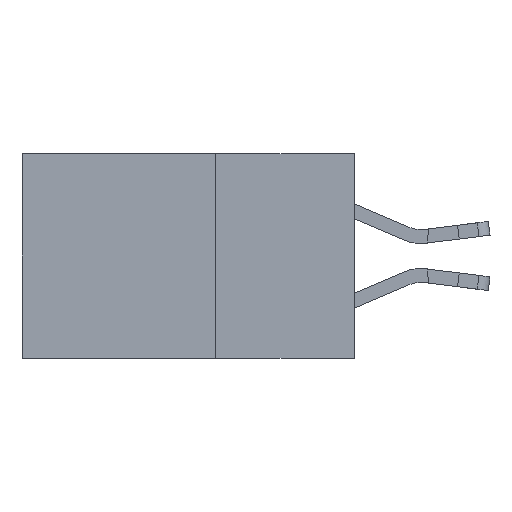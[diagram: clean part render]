
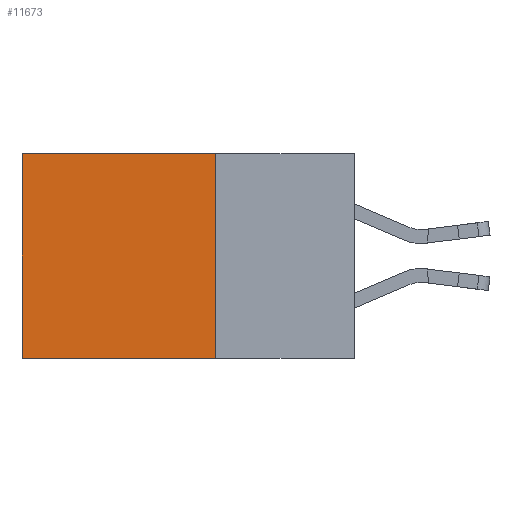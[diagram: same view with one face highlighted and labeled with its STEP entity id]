
A CAD part, left-side view. The second image highlights one B-rep face of the part: STEP entity #11673.
In plain terms, the highlighted planar face has unit normal (-1, 0, 0).
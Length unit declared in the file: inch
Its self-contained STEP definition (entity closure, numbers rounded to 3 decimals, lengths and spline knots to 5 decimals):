
#77 = VECTOR ( 'NONE', #8197, 39.37008 ) ;
#394 = LINE ( 'NONE', #10285, #77 ) ;
#401 = ORIENTED_EDGE ( 'NONE', *, *, #12165, .T. ) ;
#487 = DIRECTION ( 'NONE',  ( 0., 0., -1. ) ) ;
#513 = CARTESIAN_POINT ( 'NONE',  ( 0.298, 0.6, -0.37 ) ) ;
#648 = VERTEX_POINT ( 'NONE', #13406 ) ;
#827 = CARTESIAN_POINT ( 'NONE',  ( 0.298, 0.25, -0.37 ) ) ;
#1503 = LINE ( 'NONE', #11725, #6780 ) ;
#2200 = LINE ( 'NONE', #4501, #4677 ) ;
#2387 = DIRECTION ( 'NONE',  ( 0., 1., 0. ) ) ;
#2660 = VECTOR ( 'NONE', #4953, 39.37008 ) ;
#2956 = CARTESIAN_POINT ( 'NONE',  ( 0.298, 0.6, 0. ) ) ;
#3911 = CARTESIAN_POINT ( 'NONE',  ( 0.298, 0.6, 0. ) ) ;
#4501 = CARTESIAN_POINT ( 'NONE',  ( 0.298, 0.25, -0.37 ) ) ;
#4677 = VECTOR ( 'NONE', #10721, 39.37008 ) ;
#4953 = DIRECTION ( 'NONE',  ( 0., 0., -1. ) ) ;
#5388 = VERTEX_POINT ( 'NONE', #513 ) ;
#5645 = EDGE_CURVE ( 'NONE', #648, #9075, #394, .T. ) ;
#6734 = EDGE_CURVE ( 'NONE', #9078, #5388, #10947, .T. ) ;
#6763 = DIRECTION ( 'NONE',  ( 1., 0., 0. ) ) ;
#6780 = VECTOR ( 'NONE', #2387, 39.37008 ) ;
#6796 = FACE_OUTER_BOUND ( 'NONE', #10290, .T. ) ;
#8197 = DIRECTION ( 'NONE',  ( 0., 0., -1. ) ) ;
#9075 = VERTEX_POINT ( 'NONE', #827 ) ;
#9078 = VERTEX_POINT ( 'NONE', #2956 ) ;
#10192 = ORIENTED_EDGE ( 'NONE', *, *, #10984, .F. ) ;
#10285 = CARTESIAN_POINT ( 'NONE',  ( 0.298, 0.25, 0. ) ) ;
#10290 = EDGE_LOOP ( 'NONE', ( #13050, #10192, #12900, #401 ) ) ;
#10721 = DIRECTION ( 'NONE',  ( 0., 1., 0. ) ) ;
#10947 = LINE ( 'NONE', #3911, #2660 ) ;
#10984 = EDGE_CURVE ( 'NONE', #9075, #5388, #2200, .T. ) ;
#11673 = ADVANCED_FACE ( 'NONE', ( #6796 ), #11889, .F. ) ;
#11725 = CARTESIAN_POINT ( 'NONE',  ( 0.298, 0.25, 0. ) ) ;
#11889 = PLANE ( 'NONE',  #12934 ) ;
#12165 = EDGE_CURVE ( 'NONE', #648, #9078, #1503, .T. ) ;
#12900 = ORIENTED_EDGE ( 'NONE', *, *, #5645, .F. ) ;
#12920 = CARTESIAN_POINT ( 'NONE',  ( 0.298, 0.25, 0. ) ) ;
#12934 = AXIS2_PLACEMENT_3D ( 'NONE', #12920, #6763, #487 ) ;
#13050 = ORIENTED_EDGE ( 'NONE', *, *, #6734, .T. ) ;
#13406 = CARTESIAN_POINT ( 'NONE',  ( 0.298, 0.25, 0. ) ) ;
